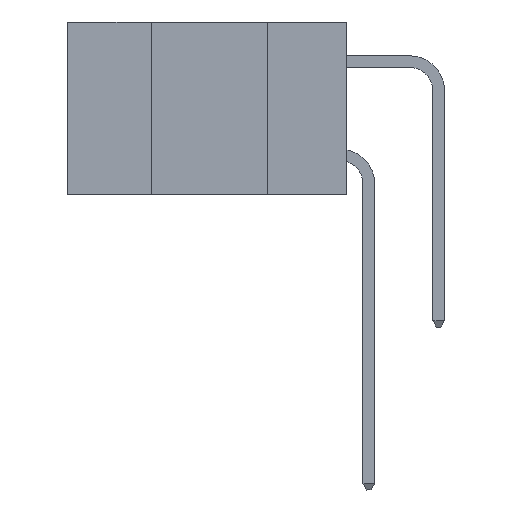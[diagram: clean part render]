
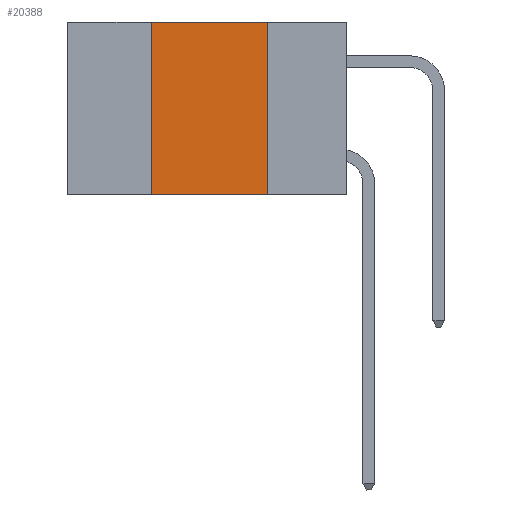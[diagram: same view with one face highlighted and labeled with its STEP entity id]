
A CAD part, left-side view. The second image highlights one B-rep face of the part: STEP entity #20388.
In plain terms, the highlighted planar face has unit normal (-1, 0, 0).
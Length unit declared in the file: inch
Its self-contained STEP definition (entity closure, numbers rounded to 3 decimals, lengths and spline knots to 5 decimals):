
#639 = CARTESIAN_POINT ( 'NONE',  ( 0., 0.6, -0.37 ) ) ;
#832 = ORIENTED_EDGE ( 'NONE', *, *, #11671, .T. ) ;
#1261 = EDGE_CURVE ( 'NONE', #21036, #9900, #4955, .T. ) ;
#1480 = LINE ( 'NONE', #10110, #19296 ) ;
#2335 = DIRECTION ( 'NONE',  ( 0., -1., 0. ) ) ;
#2779 = VECTOR ( 'NONE', #8175, 39.37008 ) ;
#2980 = EDGE_CURVE ( 'NONE', #15953, #21036, #7822, .T. ) ;
#3052 = EDGE_LOOP ( 'NONE', ( #7869, #5584, #16485, #832 ) ) ;
#3579 = DIRECTION ( 'NONE',  ( 0., -1., 0. ) ) ;
#3890 = CARTESIAN_POINT ( 'NONE',  ( 0., 0.42, -0.37 ) ) ;
#4955 = LINE ( 'NONE', #20217, #13856 ) ;
#5078 = DIRECTION ( 'NONE',  ( 0., 0., -1. ) ) ;
#5584 = ORIENTED_EDGE ( 'NONE', *, *, #1261, .F. ) ;
#5717 = AXIS2_PLACEMENT_3D ( 'NONE', #10950, #19271, #9342 ) ;
#7298 = FACE_OUTER_BOUND ( 'NONE', #3052, .T. ) ;
#7626 = PLANE ( 'NONE',  #5717 ) ;
#7822 = LINE ( 'NONE', #16492, #2779 ) ;
#7869 = ORIENTED_EDGE ( 'NONE', *, *, #15436, .F. ) ;
#8175 = DIRECTION ( 'NONE',  ( 0., 0., 1. ) ) ;
#9342 = DIRECTION ( 'NONE',  ( 0., 0., -1. ) ) ;
#9900 = VERTEX_POINT ( 'NONE', #12640 ) ;
#10110 = CARTESIAN_POINT ( 'NONE',  ( 0., 0.17, 0. ) ) ;
#10644 = VERTEX_POINT ( 'NONE', #19354 ) ;
#10950 = CARTESIAN_POINT ( 'NONE',  ( 0., 0.6, 0. ) ) ;
#11671 = EDGE_CURVE ( 'NONE', #15953, #10644, #21552, .T. ) ;
#12640 = CARTESIAN_POINT ( 'NONE',  ( 0., 0.17, 0. ) ) ;
#13856 = VECTOR ( 'NONE', #3579, 39.37008 ) ;
#15436 = EDGE_CURVE ( 'NONE', #9900, #10644, #1480, .T. ) ;
#15953 = VERTEX_POINT ( 'NONE', #3890 ) ;
#16485 = ORIENTED_EDGE ( 'NONE', *, *, #2980, .F. ) ;
#16492 = CARTESIAN_POINT ( 'NONE',  ( 0., 0.42, 0. ) ) ;
#17194 = VECTOR ( 'NONE', #2335, 39.37008 ) ;
#19271 = DIRECTION ( 'NONE',  ( 1., 0., 0. ) ) ;
#19296 = VECTOR ( 'NONE', #5078, 39.37008 ) ;
#19354 = CARTESIAN_POINT ( 'NONE',  ( 0., 0.17, -0.37 ) ) ;
#20217 = CARTESIAN_POINT ( 'NONE',  ( 0., 0.6, 0. ) ) ;
#20388 = ADVANCED_FACE ( 'NONE', ( #7298 ), #7626, .F. ) ;
#20821 = CARTESIAN_POINT ( 'NONE',  ( 0., 0.42, 0. ) ) ;
#21036 = VERTEX_POINT ( 'NONE', #20821 ) ;
#21552 = LINE ( 'NONE', #639, #17194 ) ;
